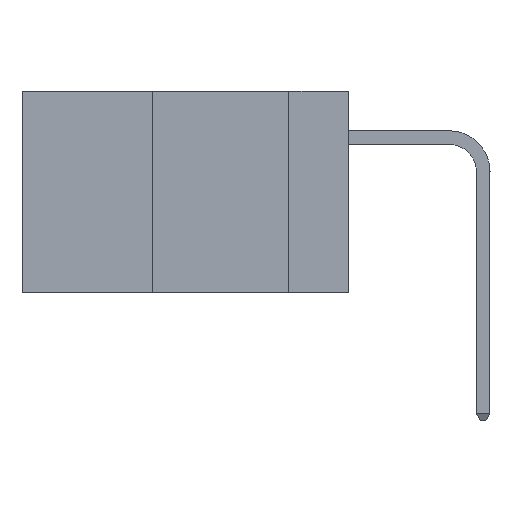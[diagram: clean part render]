
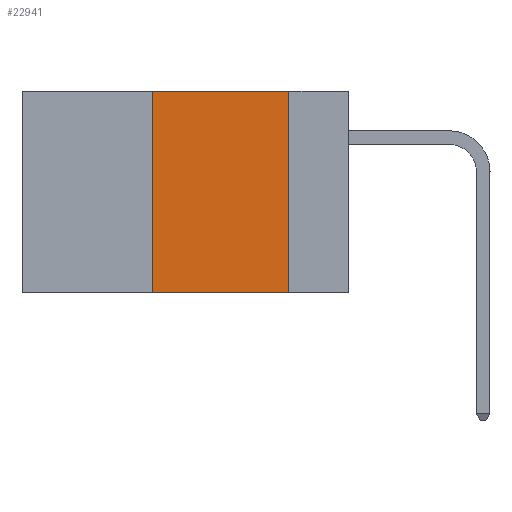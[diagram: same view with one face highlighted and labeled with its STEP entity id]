
A CAD part, left-side view. The second image highlights one B-rep face of the part: STEP entity #22941.
In plain terms, the highlighted planar face has unit normal (-1, 0, 0).
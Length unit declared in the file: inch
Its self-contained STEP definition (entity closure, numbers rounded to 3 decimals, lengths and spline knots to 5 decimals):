
#1695 = VERTEX_POINT ( 'NONE', #39364 ) ;
#2439 = DIRECTION ( 'NONE',  ( 0., 0., 1. ) ) ;
#2731 = DIRECTION ( 'NONE',  ( 0., -1., 0. ) ) ;
#4055 = ORIENTED_EDGE ( 'NONE', *, *, #42542, .T. ) ;
#5137 = DIRECTION ( 'NONE',  ( 0., -1., 0. ) ) ;
#5448 = CARTESIAN_POINT ( 'NONE',  ( 0., 0.6, 0. ) ) ;
#6403 = ORIENTED_EDGE ( 'NONE', *, *, #28244, .F. ) ;
#7092 = VECTOR ( 'NONE', #35620, 39.37008 ) ;
#9698 = DIRECTION ( 'NONE',  ( 0., 0., -1. ) ) ;
#10164 = VERTEX_POINT ( 'NONE', #22533 ) ;
#11764 = CARTESIAN_POINT ( 'NONE',  ( 0., 0.11, 0. ) ) ;
#12620 = LINE ( 'NONE', #33667, #31665 ) ;
#12740 = EDGE_CURVE ( 'NONE', #48758, #22127, #29629, .T. ) ;
#20802 = FACE_OUTER_BOUND ( 'NONE', #23855, .T. ) ;
#21887 = CARTESIAN_POINT ( 'NONE',  ( 0., 0.36, 0. ) ) ;
#22127 = VERTEX_POINT ( 'NONE', #21887 ) ;
#22533 = CARTESIAN_POINT ( 'NONE',  ( 0., 0.11, 0. ) ) ;
#22941 = ADVANCED_FACE ( 'NONE', ( #20802 ), #23440, .F. ) ;
#23440 = PLANE ( 'NONE',  #29261 ) ;
#23855 = EDGE_LOOP ( 'NONE', ( #6403, #38095, #40560, #4055 ) ) ;
#24386 = DIRECTION ( 'NONE',  ( 1., 0., 0. ) ) ;
#25814 = LINE ( 'NONE', #5448, #43605 ) ;
#28244 = EDGE_CURVE ( 'NONE', #10164, #1695, #35375, .T. ) ;
#29261 = AXIS2_PLACEMENT_3D ( 'NONE', #35587, #24386, #9698 ) ;
#29629 = LINE ( 'NONE', #45744, #50518 ) ;
#31665 = VECTOR ( 'NONE', #2731, 39.37008 ) ;
#33667 = CARTESIAN_POINT ( 'NONE',  ( 0., 0.6, -0.37 ) ) ;
#35375 = LINE ( 'NONE', #11764, #7092 ) ;
#35550 = CARTESIAN_POINT ( 'NONE',  ( 0., 0.36, -0.37 ) ) ;
#35587 = CARTESIAN_POINT ( 'NONE',  ( 0., 0.6, 0. ) ) ;
#35620 = DIRECTION ( 'NONE',  ( 0., 0., -1. ) ) ;
#38095 = ORIENTED_EDGE ( 'NONE', *, *, #47042, .F. ) ;
#39364 = CARTESIAN_POINT ( 'NONE',  ( 0., 0.11, -0.37 ) ) ;
#40560 = ORIENTED_EDGE ( 'NONE', *, *, #12740, .F. ) ;
#42542 = EDGE_CURVE ( 'NONE', #48758, #1695, #12620, .T. ) ;
#43605 = VECTOR ( 'NONE', #5137, 39.37008 ) ;
#45744 = CARTESIAN_POINT ( 'NONE',  ( 0., 0.36, 0. ) ) ;
#47042 = EDGE_CURVE ( 'NONE', #22127, #10164, #25814, .T. ) ;
#48758 = VERTEX_POINT ( 'NONE', #35550 ) ;
#50518 = VECTOR ( 'NONE', #2439, 39.37008 ) ;
